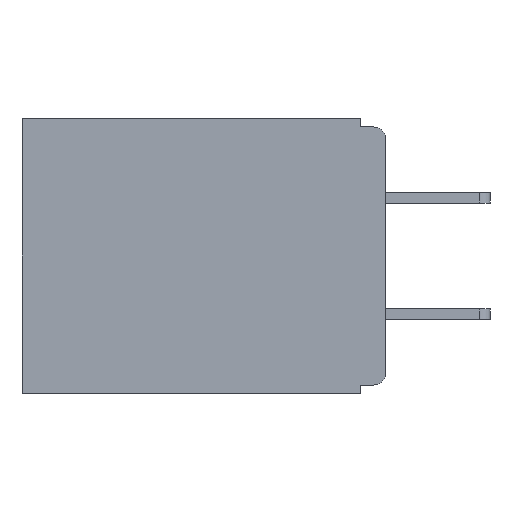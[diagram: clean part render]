
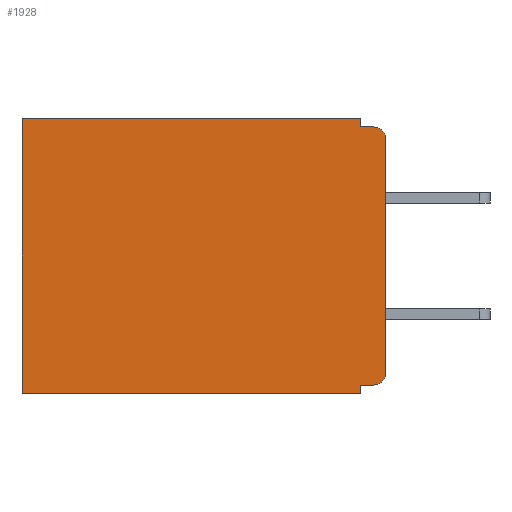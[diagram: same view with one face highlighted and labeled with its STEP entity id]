
A CAD part, left-side view. The second image highlights one B-rep face of the part: STEP entity #1928.
In plain terms, the highlighted planar face has unit normal (-1, 0, 0).
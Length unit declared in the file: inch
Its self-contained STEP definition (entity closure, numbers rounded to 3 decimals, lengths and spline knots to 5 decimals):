
#290 = CIRCLE ( 'NONE', #3081, 0.015 ) ;
#452 = ORIENTED_EDGE ( 'NONE', *, *, #2639, .F. ) ;
#769 = ORIENTED_EDGE ( 'NONE', *, *, #10743, .T. ) ;
#771 = EDGE_CURVE ( 'NONE', #5910, #6392, #9669, .T. ) ;
#805 = ORIENTED_EDGE ( 'NONE', *, *, #1619, .T. ) ;
#846 = CARTESIAN_POINT ( 'NONE',  ( 0.3, 0.437, -0.33 ) ) ;
#914 = DIRECTION ( 'NONE',  ( 1., 0., 0. ) ) ;
#1016 = ORIENTED_EDGE ( 'NONE', *, *, #1448, .F. ) ;
#1220 = LINE ( 'NONE', #8439, #9807 ) ;
#1363 = LINE ( 'NONE', #1692, #4575 ) ;
#1448 = EDGE_CURVE ( 'NONE', #6392, #1883, #8170, .T. ) ;
#1549 = ORIENTED_EDGE ( 'NONE', *, *, #771, .F. ) ;
#1619 = EDGE_CURVE ( 'NONE', #10420, #1883, #11522, .T. ) ;
#1692 = CARTESIAN_POINT ( 'NONE',  ( 0.3, 0., 0. ) ) ;
#1694 = DIRECTION ( 'NONE',  ( 0., 0., -1. ) ) ;
#1883 = VERTEX_POINT ( 'NONE', #3926 ) ;
#1928 = ADVANCED_FACE ( 'NONE', ( #5958 ), #10871, .F. ) ;
#1942 = ORIENTED_EDGE ( 'NONE', *, *, #11689, .F. ) ;
#2073 = ORIENTED_EDGE ( 'NONE', *, *, #8452, .T. ) ;
#2274 = CARTESIAN_POINT ( 'NONE',  ( 0.3, 0., -0.305 ) ) ;
#2416 = VECTOR ( 'NONE', #8637, 39.37008 ) ;
#2465 = CARTESIAN_POINT ( 'NONE',  ( 0.3, 0.015, -0.32 ) ) ;
#2639 = EDGE_CURVE ( 'NONE', #11217, #3365, #1220, .T. ) ;
#2817 = EDGE_LOOP ( 'NONE', ( #3344, #3566, #6667, #452, #769, #805, #1016, #1549, #1942, #2073 ) ) ;
#2942 = EDGE_CURVE ( 'NONE', #6356, #8135, #290, .T. ) ;
#3081 = AXIS2_PLACEMENT_3D ( 'NONE', #8128, #8102, #8161 ) ;
#3344 = ORIENTED_EDGE ( 'NONE', *, *, #11308, .F. ) ;
#3365 = VERTEX_POINT ( 'NONE', #9451 ) ;
#3371 = DIRECTION ( 'NONE',  ( 0., -1., 0. ) ) ;
#3388 = AXIS2_PLACEMENT_3D ( 'NONE', #4740, #12243, #5802 ) ;
#3566 = ORIENTED_EDGE ( 'NONE', *, *, #2942, .T. ) ;
#3709 = CARTESIAN_POINT ( 'NONE',  ( 0.3, 0., -0.33 ) ) ;
#3926 = CARTESIAN_POINT ( 'NONE',  ( 0.3, 0.437, -0.33 ) ) ;
#4258 = CARTESIAN_POINT ( 'NONE',  ( 0.3, 0., -0.025 ) ) ;
#4575 = VECTOR ( 'NONE', #9132, 39.37008 ) ;
#4740 = CARTESIAN_POINT ( 'NONE',  ( 0.3, 0.015, -0.305 ) ) ;
#5210 = DIRECTION ( 'NONE',  ( 0., 0., -1. ) ) ;
#5246 = CARTESIAN_POINT ( 'NONE',  ( 0.3, 0.015, -0.01 ) ) ;
#5384 = CARTESIAN_POINT ( 'NONE',  ( 0.3, 0.031, -0.33 ) ) ;
#5513 = LINE ( 'NONE', #10803, #8034 ) ;
#5802 = DIRECTION ( 'NONE',  ( 0., 0., -1. ) ) ;
#5910 = VERTEX_POINT ( 'NONE', #11047 ) ;
#5958 = FACE_OUTER_BOUND ( 'NONE', #2817, .T. ) ;
#6043 = LINE ( 'NONE', #9035, #13855 ) ;
#6356 = VERTEX_POINT ( 'NONE', #4258 ) ;
#6365 = LINE ( 'NONE', #11837, #2416 ) ;
#6392 = VERTEX_POINT ( 'NONE', #5384 ) ;
#6667 = ORIENTED_EDGE ( 'NONE', *, *, #12383, .F. ) ;
#7151 = VECTOR ( 'NONE', #12238, 39.37008 ) ;
#7253 = CARTESIAN_POINT ( 'NONE',  ( 0.3, 0., -0.33 ) ) ;
#7766 = DIRECTION ( 'NONE',  ( 0., 1., 0. ) ) ;
#7822 = VECTOR ( 'NONE', #7766, 39.37008 ) ;
#7929 = DIRECTION ( 'NONE',  ( 0., 0., -1. ) ) ;
#8034 = VECTOR ( 'NONE', #3371, 39.37008 ) ;
#8102 = DIRECTION ( 'NONE',  ( -1., 0., 0. ) ) ;
#8128 = CARTESIAN_POINT ( 'NONE',  ( 0.3, 0.015, -0.025 ) ) ;
#8135 = VERTEX_POINT ( 'NONE', #5246 ) ;
#8161 = DIRECTION ( 'NONE',  ( 0., 0., -1. ) ) ;
#8170 = LINE ( 'NONE', #3709, #7822 ) ;
#8439 = CARTESIAN_POINT ( 'NONE',  ( 0.3, 0.031, 0. ) ) ;
#8452 = EDGE_CURVE ( 'NONE', #11197, #10443, #8485, .T. ) ;
#8485 = CIRCLE ( 'NONE', #3388, 0.015 ) ;
#8637 = DIRECTION ( 'NONE',  ( 0., 1., 0. ) ) ;
#8682 = DIRECTION ( 'NONE',  ( 0., 0., -1. ) ) ;
#9035 = CARTESIAN_POINT ( 'NONE',  ( 0.3, 0., -0.33 ) ) ;
#9132 = DIRECTION ( 'NONE',  ( 0., 1., 0. ) ) ;
#9451 = CARTESIAN_POINT ( 'NONE',  ( 0.3, 0.031, -0.01 ) ) ;
#9669 = LINE ( 'NONE', #13085, #7151 ) ;
#9742 = CARTESIAN_POINT ( 'NONE',  ( 0.3, 0.437, 0. ) ) ;
#9807 = VECTOR ( 'NONE', #8682, 39.37008 ) ;
#10420 = VERTEX_POINT ( 'NONE', #9742 ) ;
#10443 = VERTEX_POINT ( 'NONE', #2274 ) ;
#10743 = EDGE_CURVE ( 'NONE', #11217, #10420, #1363, .T. ) ;
#10803 = CARTESIAN_POINT ( 'NONE',  ( 0.3, 0., -0.01 ) ) ;
#10871 = PLANE ( 'NONE',  #12711 ) ;
#11046 = CARTESIAN_POINT ( 'NONE',  ( 0.3, 0.031, 0. ) ) ;
#11047 = CARTESIAN_POINT ( 'NONE',  ( 0.3, 0.031, -0.32 ) ) ;
#11197 = VERTEX_POINT ( 'NONE', #2465 ) ;
#11217 = VERTEX_POINT ( 'NONE', #11046 ) ;
#11308 = EDGE_CURVE ( 'NONE', #6356, #10443, #6043, .T. ) ;
#11522 = LINE ( 'NONE', #846, #11717 ) ;
#11689 = EDGE_CURVE ( 'NONE', #11197, #5910, #6365, .T. ) ;
#11717 = VECTOR ( 'NONE', #5210, 39.37008 ) ;
#11837 = CARTESIAN_POINT ( 'NONE',  ( 0.3, 0., -0.32 ) ) ;
#12238 = DIRECTION ( 'NONE',  ( 0., 0., -1. ) ) ;
#12243 = DIRECTION ( 'NONE',  ( -1., 0., 0. ) ) ;
#12383 = EDGE_CURVE ( 'NONE', #3365, #8135, #5513, .T. ) ;
#12711 = AXIS2_PLACEMENT_3D ( 'NONE', #7253, #914, #1694 ) ;
#13085 = CARTESIAN_POINT ( 'NONE',  ( 0.3, 0.031, -0.33 ) ) ;
#13855 = VECTOR ( 'NONE', #7929, 39.37008 ) ;
